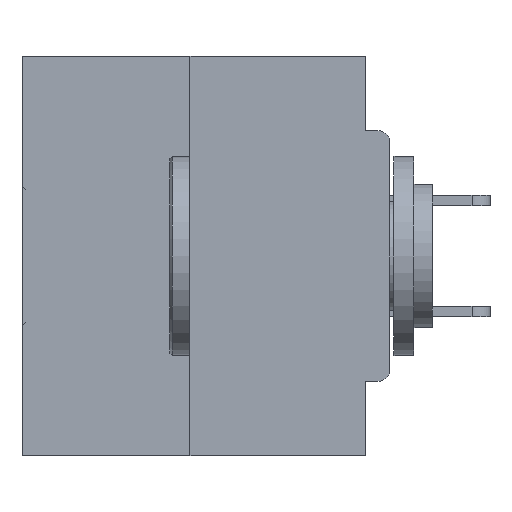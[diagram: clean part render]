
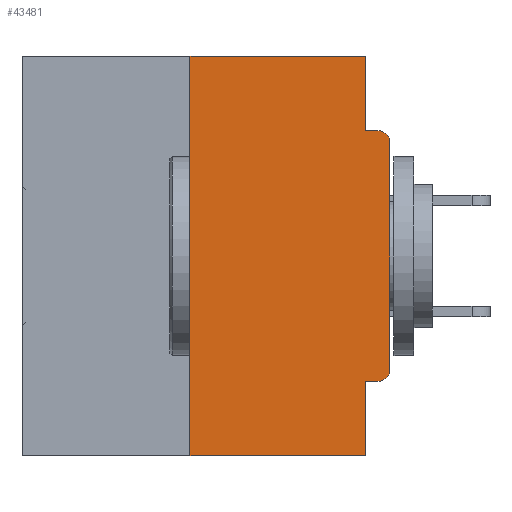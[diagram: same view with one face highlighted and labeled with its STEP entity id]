
A CAD part, left-side view. The second image highlights one B-rep face of the part: STEP entity #43481.
In plain terms, the highlighted planar face has unit normal (-1, 0, 0).
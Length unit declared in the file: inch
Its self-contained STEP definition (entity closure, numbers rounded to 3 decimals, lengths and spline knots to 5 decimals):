
#149 = VERTEX_POINT ( 'NONE', #26734 ) ;
#237 = VECTOR ( 'NONE', #37260, 39.37008 ) ;
#426 = LINE ( 'NONE', #5386, #31942 ) ;
#548 = LINE ( 'NONE', #24531, #35736 ) ;
#1343 = VERTEX_POINT ( 'NONE', #27414 ) ;
#1489 = VERTEX_POINT ( 'NONE', #41631 ) ;
#1514 = DIRECTION ( 'NONE',  ( 0., 0., -1. ) ) ;
#1686 = AXIS2_PLACEMENT_3D ( 'NONE', #36517, #9785, #37102 ) ;
#2568 = CIRCLE ( 'NONE', #38249, 0.015 ) ;
#3810 = DIRECTION ( 'NONE',  ( 0., 0., -1. ) ) ;
#5386 = CARTESIAN_POINT ( 'NONE',  ( 0., 0.031, -0.5 ) ) ;
#5502 = CARTESIAN_POINT ( 'NONE',  ( 0., 0., -0.4065 ) ) ;
#5651 = DIRECTION ( 'NONE',  ( 0., 0., -1. ) ) ;
#5658 = ORIENTED_EDGE ( 'NONE', *, *, #31210, .F. ) ;
#6426 = CARTESIAN_POINT ( 'NONE',  ( 0., 0.015, -0.1085 ) ) ;
#7297 = CARTESIAN_POINT ( 'NONE',  ( 0., 0., 0. ) ) ;
#8023 = CARTESIAN_POINT ( 'NONE',  ( 0., 0., -0.3915 ) ) ;
#9648 = PLANE ( 'NONE',  #1686 ) ;
#9785 = DIRECTION ( 'NONE',  ( 1., 0., 0. ) ) ;
#9844 = EDGE_CURVE ( 'NONE', #36594, #41317, #426, .T. ) ;
#10300 = VERTEX_POINT ( 'NONE', #8023 ) ;
#10346 = VERTEX_POINT ( 'NONE', #41659 ) ;
#10478 = ORIENTED_EDGE ( 'NONE', *, *, #29145, .F. ) ;
#10990 = EDGE_LOOP ( 'NONE', ( #5658, #15194, #25957, #12330, #10478, #19245, #35863, #35393, #38883, #16740 ) ) ;
#11339 = CARTESIAN_POINT ( 'NONE',  ( 0., 0.25, 0. ) ) ;
#12330 = ORIENTED_EDGE ( 'NONE', *, *, #9844, .F. ) ;
#13009 = VECTOR ( 'NONE', #35495, 39.37008 ) ;
#15194 = ORIENTED_EDGE ( 'NONE', *, *, #29831, .F. ) ;
#15327 = CARTESIAN_POINT ( 'NONE',  ( 0., 0.015, -0.3915 ) ) ;
#15510 = DIRECTION ( 'NONE',  ( 0., -1., 0. ) ) ;
#15560 = EDGE_CURVE ( 'NONE', #37730, #40413, #548, .T. ) ;
#15711 = VECTOR ( 'NONE', #27624, 39.37008 ) ;
#16014 = EDGE_CURVE ( 'NONE', #1343, #149, #29888, .T. ) ;
#16250 = CARTESIAN_POINT ( 'NONE',  ( 0., 0.031, 0. ) ) ;
#16575 = LINE ( 'NONE', #7297, #237 ) ;
#16740 = ORIENTED_EDGE ( 'NONE', *, *, #15560, .F. ) ;
#17292 = LINE ( 'NONE', #23792, #15711 ) ;
#17499 = FACE_OUTER_BOUND ( 'NONE', #10990, .T. ) ;
#17945 = CARTESIAN_POINT ( 'NONE',  ( 0., 0.031, -0.0935 ) ) ;
#17986 = VECTOR ( 'NONE', #15510, 39.37008 ) ;
#18084 = DIRECTION ( 'NONE',  ( 0., 0., 1. ) ) ;
#18702 = DIRECTION ( 'NONE',  ( -1., 0., 0. ) ) ;
#19162 = CARTESIAN_POINT ( 'NONE',  ( 0., 0., -0.0935 ) ) ;
#19245 = ORIENTED_EDGE ( 'NONE', *, *, #19834, .T. ) ;
#19834 = EDGE_CURVE ( 'NONE', #10346, #10300, #2568, .T. ) ;
#21129 = LINE ( 'NONE', #19162, #17986 ) ;
#22909 = DIRECTION ( 'NONE',  ( 0., 0., -1. ) ) ;
#23792 = CARTESIAN_POINT ( 'NONE',  ( 0., 0.46, 0. ) ) ;
#24531 = CARTESIAN_POINT ( 'NONE',  ( 0., 0.031, 0. ) ) ;
#24606 = EDGE_CURVE ( 'NONE', #10300, #1343, #16575, .T. ) ;
#24899 = CARTESIAN_POINT ( 'NONE',  ( 0., 0.46, -0.5 ) ) ;
#25474 = VECTOR ( 'NONE', #34738, 39.37008 ) ;
#25957 = ORIENTED_EDGE ( 'NONE', *, *, #38680, .T. ) ;
#26013 = EDGE_CURVE ( 'NONE', #40413, #149, #21129, .T. ) ;
#26104 = CARTESIAN_POINT ( 'NONE',  ( 0., 0.25, 0. ) ) ;
#26734 = CARTESIAN_POINT ( 'NONE',  ( 0., 0.015, -0.0935 ) ) ;
#27131 = LINE ( 'NONE', #11339, #29188 ) ;
#27414 = CARTESIAN_POINT ( 'NONE',  ( 0., 0., -0.1085 ) ) ;
#27624 = DIRECTION ( 'NONE',  ( 0., -1., 0. ) ) ;
#29145 = EDGE_CURVE ( 'NONE', #10346, #36594, #37180, .T. ) ;
#29188 = VECTOR ( 'NONE', #18084, 39.37008 ) ;
#29831 = EDGE_CURVE ( 'NONE', #1489, #42758, #27131, .T. ) ;
#29888 = CIRCLE ( 'NONE', #33687, 0.015 ) ;
#29921 = DIRECTION ( 'NONE',  ( -1., 0., 0. ) ) ;
#30677 = CARTESIAN_POINT ( 'NONE',  ( 0., 0.031, -0.5 ) ) ;
#31210 = EDGE_CURVE ( 'NONE', #42758, #37730, #17292, .T. ) ;
#31942 = VECTOR ( 'NONE', #5651, 39.37008 ) ;
#33687 = AXIS2_PLACEMENT_3D ( 'NONE', #6426, #29921, #22909 ) ;
#34284 = CARTESIAN_POINT ( 'NONE',  ( 0., 0.031, -0.4065 ) ) ;
#34738 = DIRECTION ( 'NONE',  ( 0., -1., 0. ) ) ;
#35393 = ORIENTED_EDGE ( 'NONE', *, *, #16014, .T. ) ;
#35495 = DIRECTION ( 'NONE',  ( 0., 1., 0. ) ) ;
#35736 = VECTOR ( 'NONE', #3810, 39.37008 ) ;
#35863 = ORIENTED_EDGE ( 'NONE', *, *, #24606, .T. ) ;
#36517 = CARTESIAN_POINT ( 'NONE',  ( 0., 0.46, 0. ) ) ;
#36594 = VERTEX_POINT ( 'NONE', #34284 ) ;
#37102 = DIRECTION ( 'NONE',  ( 0., 0., -1. ) ) ;
#37180 = LINE ( 'NONE', #5502, #13009 ) ;
#37260 = DIRECTION ( 'NONE',  ( 0., 0., 1. ) ) ;
#37730 = VERTEX_POINT ( 'NONE', #16250 ) ;
#38249 = AXIS2_PLACEMENT_3D ( 'NONE', #15327, #18702, #1514 ) ;
#38680 = EDGE_CURVE ( 'NONE', #1489, #41317, #41795, .T. ) ;
#38883 = ORIENTED_EDGE ( 'NONE', *, *, #26013, .F. ) ;
#40413 = VERTEX_POINT ( 'NONE', #17945 ) ;
#41317 = VERTEX_POINT ( 'NONE', #30677 ) ;
#41631 = CARTESIAN_POINT ( 'NONE',  ( 0., 0.25, -0.5 ) ) ;
#41659 = CARTESIAN_POINT ( 'NONE',  ( 0., 0.015, -0.4065 ) ) ;
#41795 = LINE ( 'NONE', #24899, #25474 ) ;
#42758 = VERTEX_POINT ( 'NONE', #26104 ) ;
#43481 = ADVANCED_FACE ( 'NONE', ( #17499 ), #9648, .F. ) ;
